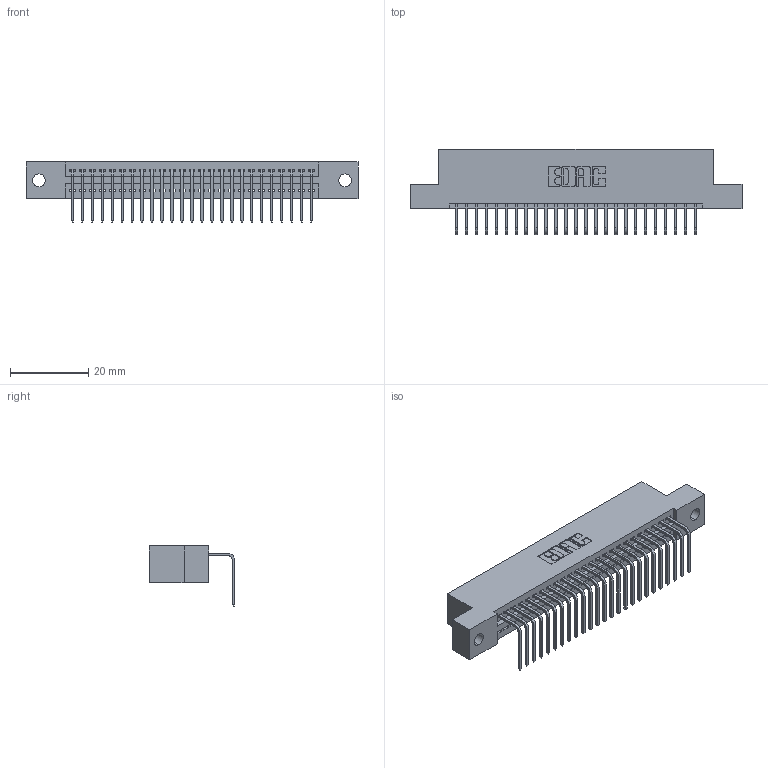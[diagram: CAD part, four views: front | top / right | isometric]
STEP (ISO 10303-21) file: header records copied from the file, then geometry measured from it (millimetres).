
FILE_DESCRIPTION (( 'STEP AP203' ), '1' );
FILE_NAME ('395-025-558-102.STEP', '2019-10-11T04:59:36', ( '' ), ( '' ), 'SwSTEP 2.0', 'SolidWorks 2016', '' );
FILE_SCHEMA (( 'CONFIG_CONTROL_DESIGN' ));
Length unit declared in the file: inch
Products named in the file (3): 345 Part_Flush Mounting Lugs - 0.128 Dia; 345-292-001_558 Tail - 2; 395-025-558-102
Assembly tree (26 placements, depth 2):
  395-025-558-102
    345 Part_Flush Mounting Lugs - 0.128 Dia
    345-292-001_558 Tail - 2  x25
Bounding box: 84.71 x 21.83 x 15.37 mm (x, y, z)
Volume: 7953.1 mm3; surface area: 10555.8 mm2
Topology: 26 solids, 26 shells, 1626 faces, 4891 edges, 3226 vertices
Faces by surface type: plane 1130, cylinder 496
Entity records: 21191 total; most frequent: CARTESIAN_POINT 3679, ORIENTED_EDGE 3638, DIRECTION 3237, EDGE_CURVE 1819, LINE 1587, VECTOR 1587, VERTEX_POINT 1210, AXIS2_PLACEMENT_3D 825
